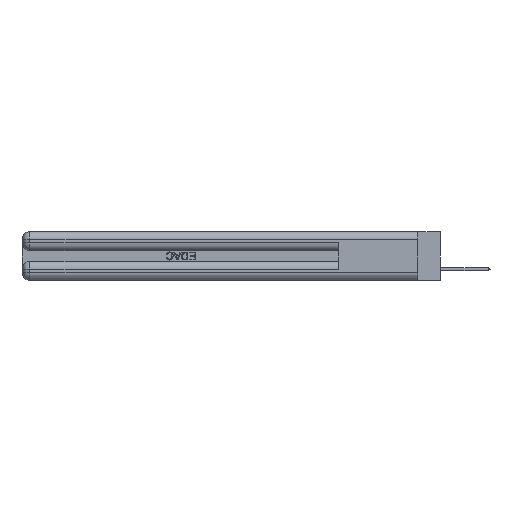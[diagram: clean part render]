
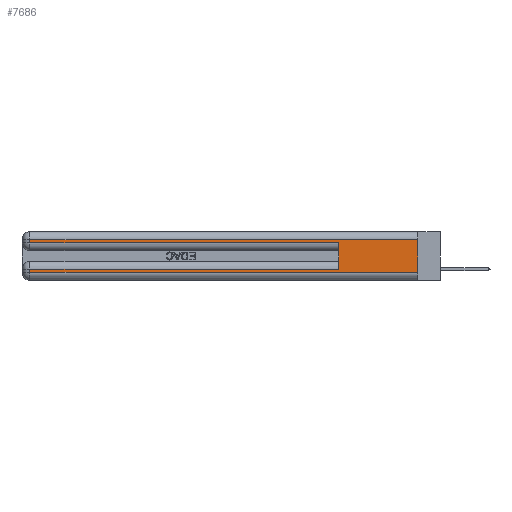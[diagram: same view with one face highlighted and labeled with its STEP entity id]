
A CAD part, left-side view. The second image highlights one B-rep face of the part: STEP entity #7686.
In plain terms, the highlighted planar face has unit normal (-1, 0, 0).
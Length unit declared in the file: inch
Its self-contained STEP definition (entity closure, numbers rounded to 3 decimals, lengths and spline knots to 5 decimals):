
#355 = LINE ( 'NONE', #18795, #18680 ) ;
#576 = VECTOR ( 'NONE', #13922, 39.37008 ) ;
#1111 = ORIENTED_EDGE ( 'NONE', *, *, #29931, .F. ) ;
#1344 = PLANE ( 'NONE',  #47113 ) ;
#1434 = DIRECTION ( 'NONE',  ( 0., 0., 1. ) ) ;
#1537 = CARTESIAN_POINT ( 'NONE',  ( 0., 2.94, 0.285 ) ) ;
#1563 = LINE ( 'NONE', #30593, #13408 ) ;
#2198 = CARTESIAN_POINT ( 'NONE',  ( 0., 0., 0.06 ) ) ;
#2318 = DIRECTION ( 'NONE',  ( 0., 1., 0. ) ) ;
#2626 = ORIENTED_EDGE ( 'NONE', *, *, #23855, .T. ) ;
#3098 = VERTEX_POINT ( 'NONE', #1537 ) ;
#3319 = VECTOR ( 'NONE', #27771, 39.37008 ) ;
#5861 = LINE ( 'NONE', #7986, #19971 ) ;
#6437 = FACE_OUTER_BOUND ( 'NONE', #25950, .T. ) ;
#7660 = ORIENTED_EDGE ( 'NONE', *, *, #26296, .T. ) ;
#7686 = ADVANCED_FACE ( 'NONE', ( #6437 ), #1344, .F. ) ;
#7986 = CARTESIAN_POINT ( 'NONE',  ( 0., 2.94, 0.37 ) ) ;
#9132 = CARTESIAN_POINT ( 'NONE',  ( 0., 0., 0.06 ) ) ;
#10560 = VECTOR ( 'NONE', #2318, 39.37008 ) ;
#10702 = LINE ( 'NONE', #2198, #576 ) ;
#11238 = DIRECTION ( 'NONE',  ( 0., 0., -1. ) ) ;
#11591 = CARTESIAN_POINT ( 'NONE',  ( 0., 0.6, 0.085 ) ) ;
#11881 = DIRECTION ( 'NONE',  ( 0., 0., -1. ) ) ;
#12208 = EDGE_CURVE ( 'NONE', #41564, #16694, #15686, .T. ) ;
#13408 = VECTOR ( 'NONE', #11238, 39.37008 ) ;
#13853 = ORIENTED_EDGE ( 'NONE', *, *, #37443, .T. ) ;
#13892 = CARTESIAN_POINT ( 'NONE',  ( 0., 0., 0.37 ) ) ;
#13922 = DIRECTION ( 'NONE',  ( 0., -1., 0. ) ) ;
#15460 = ORIENTED_EDGE ( 'NONE', *, *, #12208, .F. ) ;
#15686 = LINE ( 'NONE', #16467, #3319 ) ;
#16467 = CARTESIAN_POINT ( 'NONE',  ( 0., 0., 0.37 ) ) ;
#16694 = VERTEX_POINT ( 'NONE', #9132 ) ;
#17844 = DIRECTION ( 'NONE',  ( 1., 0., 0. ) ) ;
#18680 = VECTOR ( 'NONE', #1434, 39.37008 ) ;
#18795 = CARTESIAN_POINT ( 'NONE',  ( 0., 0.6, 0.145 ) ) ;
#19683 = ORIENTED_EDGE ( 'NONE', *, *, #39148, .T. ) ;
#19971 = VECTOR ( 'NONE', #46605, 39.37008 ) ;
#20509 = VERTEX_POINT ( 'NONE', #33151 ) ;
#20606 = VERTEX_POINT ( 'NONE', #30776 ) ;
#21152 = EDGE_CURVE ( 'NONE', #20606, #3098, #1563, .T. ) ;
#22894 = VERTEX_POINT ( 'NONE', #11591 ) ;
#22971 = ORIENTED_EDGE ( 'NONE', *, *, #38126, .T. ) ;
#23855 = EDGE_CURVE ( 'NONE', #20509, #16694, #10702, .T. ) ;
#25950 = EDGE_LOOP ( 'NONE', ( #15460, #22971, #36086, #19683, #1111, #7660, #13853, #2626 ) ) ;
#26112 = CARTESIAN_POINT ( 'NONE',  ( 0., 0., 0.285 ) ) ;
#26296 = EDGE_CURVE ( 'NONE', #22894, #39658, #39106, .T. ) ;
#26905 = CARTESIAN_POINT ( 'NONE',  ( 0., 0., 0.085 ) ) ;
#27771 = DIRECTION ( 'NONE',  ( 0., 0., -1. ) ) ;
#28009 = VECTOR ( 'NONE', #41768, 39.37008 ) ;
#29478 = CARTESIAN_POINT ( 'NONE',  ( 0., 2.94, 0.085 ) ) ;
#29551 = CARTESIAN_POINT ( 'NONE',  ( 0., 0.6, 0.285 ) ) ;
#29843 = DIRECTION ( 'NONE',  ( 0., -1., 0. ) ) ;
#29931 = EDGE_CURVE ( 'NONE', #22894, #32613, #355, .T. ) ;
#30593 = CARTESIAN_POINT ( 'NONE',  ( 0., 2.94, 0.37 ) ) ;
#30776 = CARTESIAN_POINT ( 'NONE',  ( 0., 2.94, 0.31 ) ) ;
#32085 = VECTOR ( 'NONE', #29843, 39.37008 ) ;
#32613 = VERTEX_POINT ( 'NONE', #29551 ) ;
#33151 = CARTESIAN_POINT ( 'NONE',  ( 0., 2.94, 0.06 ) ) ;
#36086 = ORIENTED_EDGE ( 'NONE', *, *, #21152, .T. ) ;
#37443 = EDGE_CURVE ( 'NONE', #39658, #20509, #5861, .T. ) ;
#38126 = EDGE_CURVE ( 'NONE', #41564, #20606, #48093, .T. ) ;
#39106 = LINE ( 'NONE', #26905, #28009 ) ;
#39148 = EDGE_CURVE ( 'NONE', #3098, #32613, #48569, .T. ) ;
#39565 = CARTESIAN_POINT ( 'NONE',  ( 0., 0., 0.31 ) ) ;
#39658 = VERTEX_POINT ( 'NONE', #29478 ) ;
#40425 = CARTESIAN_POINT ( 'NONE',  ( 0., 0., 0.31 ) ) ;
#41564 = VERTEX_POINT ( 'NONE', #40425 ) ;
#41768 = DIRECTION ( 'NONE',  ( 0., 1., 0. ) ) ;
#46605 = DIRECTION ( 'NONE',  ( 0., 0., -1. ) ) ;
#47113 = AXIS2_PLACEMENT_3D ( 'NONE', #13892, #17844, #11881 ) ;
#48093 = LINE ( 'NONE', #39565, #10560 ) ;
#48569 = LINE ( 'NONE', #26112, #32085 ) ;
